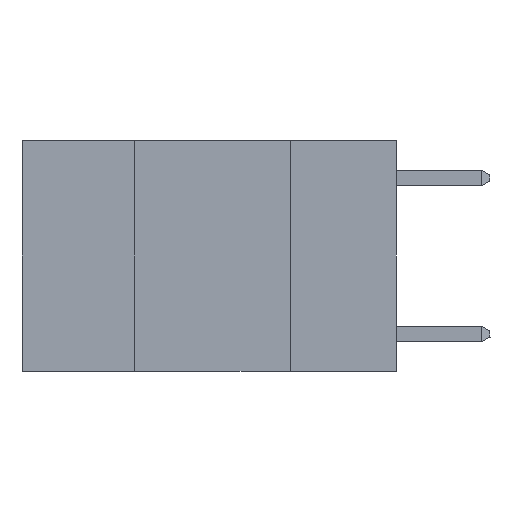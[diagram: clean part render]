
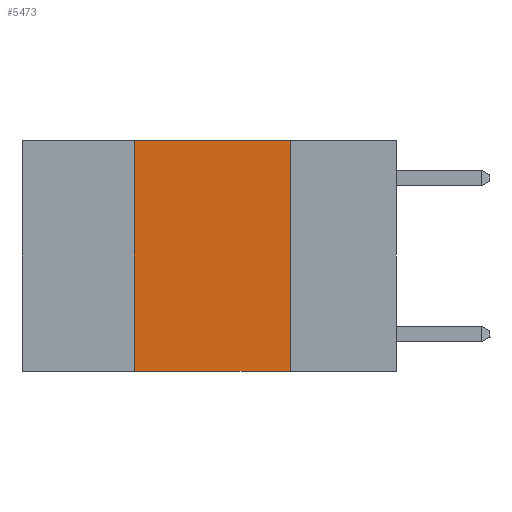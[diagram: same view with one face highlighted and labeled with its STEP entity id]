
A CAD part, left-side view. The second image highlights one B-rep face of the part: STEP entity #5473.
In plain terms, the highlighted planar face has unit normal (-1, 0, 0).
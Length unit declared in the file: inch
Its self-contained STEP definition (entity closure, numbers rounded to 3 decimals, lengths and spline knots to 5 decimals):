
#53 = CARTESIAN_POINT ( 'NONE',  ( 0., 0.42, 0. ) ) ;
#309 = FACE_OUTER_BOUND ( 'NONE', #1428, .T. ) ;
#497 = VERTEX_POINT ( 'NONE', #13032 ) ;
#1059 = DIRECTION ( 'NONE',  ( 0., -1., 0. ) ) ;
#1428 = EDGE_LOOP ( 'NONE', ( #4475, #5421, #5434, #5735 ) ) ;
#1535 = VECTOR ( 'NONE', #5480, 39.37008 ) ;
#1716 = DIRECTION ( 'NONE',  ( 1., 0., 0. ) ) ;
#1807 = EDGE_CURVE ( 'NONE', #9666, #497, #7616, .T. ) ;
#2204 = VECTOR ( 'NONE', #12779, 39.37008 ) ;
#3172 = LINE ( 'NONE', #8914, #11252 ) ;
#4337 = AXIS2_PLACEMENT_3D ( 'NONE', #6304, #1716, #9595 ) ;
#4475 = ORIENTED_EDGE ( 'NONE', *, *, #1807, .F. ) ;
#5421 = ORIENTED_EDGE ( 'NONE', *, *, #11261, .F. ) ;
#5434 = ORIENTED_EDGE ( 'NONE', *, *, #7560, .F. ) ;
#5473 = ADVANCED_FACE ( 'NONE', ( #309 ), #8523, .F. ) ;
#5480 = DIRECTION ( 'NONE',  ( 0., 0., -1. ) ) ;
#5735 = ORIENTED_EDGE ( 'NONE', *, *, #7287, .T. ) ;
#6304 = CARTESIAN_POINT ( 'NONE',  ( 0., 0.6, 0. ) ) ;
#7029 = VECTOR ( 'NONE', #10152, 39.37008 ) ;
#7130 = CARTESIAN_POINT ( 'NONE',  ( 0., 0.17, 0. ) ) ;
#7287 = EDGE_CURVE ( 'NONE', #7645, #497, #11038, .T. ) ;
#7560 = EDGE_CURVE ( 'NONE', #7645, #9155, #10215, .T. ) ;
#7616 = LINE ( 'NONE', #13979, #1535 ) ;
#7645 = VERTEX_POINT ( 'NONE', #12262 ) ;
#8523 = PLANE ( 'NONE',  #4337 ) ;
#8914 = CARTESIAN_POINT ( 'NONE',  ( 0., 0.6, 0. ) ) ;
#9155 = VERTEX_POINT ( 'NONE', #9766 ) ;
#9595 = DIRECTION ( 'NONE',  ( 0., 0., -1. ) ) ;
#9666 = VERTEX_POINT ( 'NONE', #7130 ) ;
#9766 = CARTESIAN_POINT ( 'NONE',  ( 0., 0.42, 0. ) ) ;
#10152 = DIRECTION ( 'NONE',  ( 0., 0., 1. ) ) ;
#10215 = LINE ( 'NONE', #53, #7029 ) ;
#11038 = LINE ( 'NONE', #12735, #2204 ) ;
#11252 = VECTOR ( 'NONE', #1059, 39.37008 ) ;
#11261 = EDGE_CURVE ( 'NONE', #9155, #9666, #3172, .T. ) ;
#12262 = CARTESIAN_POINT ( 'NONE',  ( 0., 0.42, -0.37 ) ) ;
#12735 = CARTESIAN_POINT ( 'NONE',  ( 0., 0.6, -0.37 ) ) ;
#12779 = DIRECTION ( 'NONE',  ( 0., -1., 0. ) ) ;
#13032 = CARTESIAN_POINT ( 'NONE',  ( 0., 0.17, -0.37 ) ) ;
#13979 = CARTESIAN_POINT ( 'NONE',  ( 0., 0.17, 0. ) ) ;
